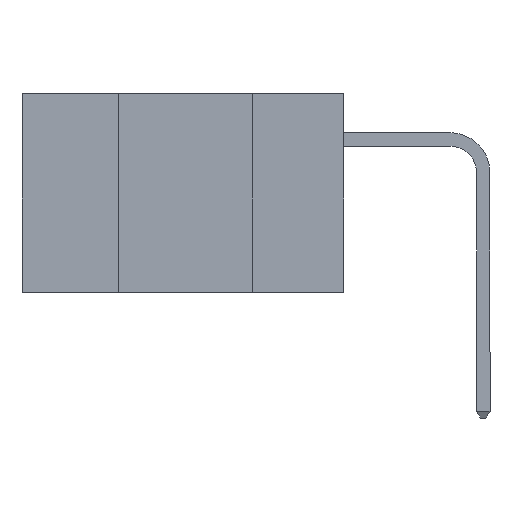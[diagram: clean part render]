
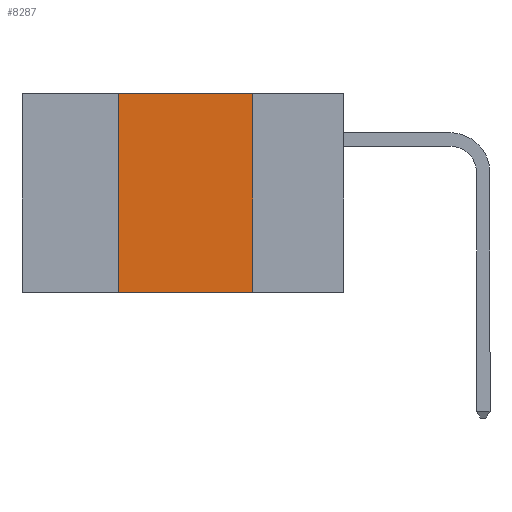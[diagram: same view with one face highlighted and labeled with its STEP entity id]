
A CAD part, left-side view. The second image highlights one B-rep face of the part: STEP entity #8287.
In plain terms, the highlighted planar face has unit normal (-1, 0, 0).
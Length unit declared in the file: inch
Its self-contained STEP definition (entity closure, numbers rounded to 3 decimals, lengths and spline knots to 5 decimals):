
#136 = VERTEX_POINT ( 'NONE', #7808 ) ;
#853 = ORIENTED_EDGE ( 'NONE', *, *, #6537, .F. ) ;
#1075 = ORIENTED_EDGE ( 'NONE', *, *, #16058, .F. ) ;
#1211 = ORIENTED_EDGE ( 'NONE', *, *, #5436, .F. ) ;
#1259 = ORIENTED_EDGE ( 'NONE', *, *, #4303, .T. ) ;
#2954 = CARTESIAN_POINT ( 'NONE',  ( 0., 0.6, 0. ) ) ;
#3715 = CARTESIAN_POINT ( 'NONE',  ( 0., 0.6, 0. ) ) ;
#3722 = AXIS2_PLACEMENT_3D ( 'NONE', #3715, #5415, #16620 ) ;
#4303 = EDGE_CURVE ( 'NONE', #13406, #136, #19288, .T. ) ;
#5132 = FACE_OUTER_BOUND ( 'NONE', #12327, .T. ) ;
#5415 = DIRECTION ( 'NONE',  ( 1., 0., 0. ) ) ;
#5436 = EDGE_CURVE ( 'NONE', #13406, #6187, #14049, .T. ) ;
#6187 = VERTEX_POINT ( 'NONE', #6979 ) ;
#6537 = EDGE_CURVE ( 'NONE', #17117, #136, #17492, .T. ) ;
#6652 = DIRECTION ( 'NONE',  ( 0., 0., 1. ) ) ;
#6979 = CARTESIAN_POINT ( 'NONE',  ( 0., 0.42, 0. ) ) ;
#7808 = CARTESIAN_POINT ( 'NONE',  ( 0., 0.17, -0.37 ) ) ;
#8287 = ADVANCED_FACE ( 'NONE', ( #5132 ), #13408, .F. ) ;
#8709 = DIRECTION ( 'NONE',  ( 0., -1., 0. ) ) ;
#9396 = VECTOR ( 'NONE', #6652, 39.37008 ) ;
#10972 = DIRECTION ( 'NONE',  ( 0., 0., -1. ) ) ;
#12327 = EDGE_LOOP ( 'NONE', ( #853, #1075, #1211, #1259 ) ) ;
#13269 = VECTOR ( 'NONE', #10972, 39.37008 ) ;
#13406 = VERTEX_POINT ( 'NONE', #15020 ) ;
#13408 = PLANE ( 'NONE',  #3722 ) ;
#14020 = VECTOR ( 'NONE', #14296, 39.37008 ) ;
#14049 = LINE ( 'NONE', #16218, #9396 ) ;
#14080 = CARTESIAN_POINT ( 'NONE',  ( 0., 0.17, 0. ) ) ;
#14296 = DIRECTION ( 'NONE',  ( 0., -1., 0. ) ) ;
#14511 = LINE ( 'NONE', #2954, #14020 ) ;
#14558 = VECTOR ( 'NONE', #8709, 39.37008 ) ;
#15020 = CARTESIAN_POINT ( 'NONE',  ( 0., 0.42, -0.37 ) ) ;
#16058 = EDGE_CURVE ( 'NONE', #6187, #17117, #14511, .T. ) ;
#16218 = CARTESIAN_POINT ( 'NONE',  ( 0., 0.42, 0. ) ) ;
#16620 = DIRECTION ( 'NONE',  ( 0., 0., -1. ) ) ;
#17117 = VERTEX_POINT ( 'NONE', #18722 ) ;
#17492 = LINE ( 'NONE', #14080, #13269 ) ;
#18189 = CARTESIAN_POINT ( 'NONE',  ( 0., 0.6, -0.37 ) ) ;
#18722 = CARTESIAN_POINT ( 'NONE',  ( 0., 0.17, 0. ) ) ;
#19288 = LINE ( 'NONE', #18189, #14558 ) ;
